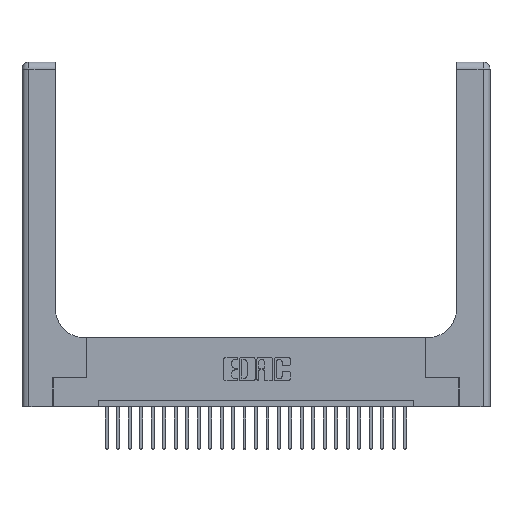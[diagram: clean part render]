
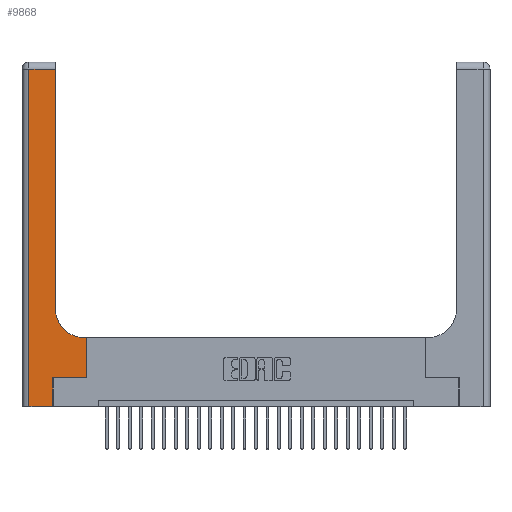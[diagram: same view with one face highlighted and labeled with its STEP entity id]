
A CAD part, top view. The second image highlights one B-rep face of the part: STEP entity #9868.
In plain terms, the highlighted planar face has unit normal (0, 0, 1).
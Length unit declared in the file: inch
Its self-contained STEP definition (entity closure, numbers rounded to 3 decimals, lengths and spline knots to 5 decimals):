
#436 = CARTESIAN_POINT ( 'NONE',  ( 0.2915, 3., 0.37 ) ) ;
#703 = DIRECTION ( 'NONE',  ( 1., 0., 0. ) ) ;
#1467 = VECTOR ( 'NONE', #26861, 39.37008 ) ;
#2086 = VECTOR ( 'NONE', #13174, 39.37008 ) ;
#2354 = CARTESIAN_POINT ( 'NONE',  ( 0.2915, 2.94, 0.37 ) ) ;
#2868 = ORIENTED_EDGE ( 'NONE', *, *, #5653, .T. ) ;
#3011 = LINE ( 'NONE', #5509, #11311 ) ;
#3412 = LINE ( 'NONE', #19778, #13361 ) ;
#3450 = LINE ( 'NONE', #25902, #2086 ) ;
#5258 = ORIENTED_EDGE ( 'NONE', *, *, #16077, .T. ) ;
#5509 = CARTESIAN_POINT ( 'NONE',  ( 0.5585, 0.25, 0.37 ) ) ;
#5653 = EDGE_CURVE ( 'NONE', #23626, #8141, #13226, .T. ) ;
#5696 = DIRECTION ( 'NONE',  ( 0., 0., -1. ) ) ;
#5724 = AXIS2_PLACEMENT_3D ( 'NONE', #27100, #14184, #27290 ) ;
#5874 = CARTESIAN_POINT ( 'NONE',  ( 0.5585, 0.6, 0.37 ) ) ;
#5972 = ORIENTED_EDGE ( 'NONE', *, *, #16115, .T. ) ;
#6153 = EDGE_CURVE ( 'NONE', #8141, #24420, #18216, .T. ) ;
#6887 = DIRECTION ( 'NONE',  ( 0., 1., 0. ) ) ;
#6962 = VERTEX_POINT ( 'NONE', #26243 ) ;
#7846 = CARTESIAN_POINT ( 'NONE',  ( 0., 2.94, 0.37 ) ) ;
#7862 = EDGE_LOOP ( 'NONE', ( #17325, #14913, #5258, #5972, #20539, #14708, #23998, #15144, #2868 ) ) ;
#8029 = CARTESIAN_POINT ( 'NONE',  ( 0.5415, 0.6, 0.37 ) ) ;
#8141 = VERTEX_POINT ( 'NONE', #10238 ) ;
#8987 = VECTOR ( 'NONE', #22697, 39.37008 ) ;
#9721 = VERTEX_POINT ( 'NONE', #13995 ) ;
#9868 = ADVANCED_FACE ( 'NONE', ( #16337 ), #20171, .F. ) ;
#9950 = CARTESIAN_POINT ( 'NONE',  ( 0.2915, 0.6, 0.37 ) ) ;
#10238 = CARTESIAN_POINT ( 'NONE',  ( 0.2915, 0.85, 0.37 ) ) ;
#10273 = EDGE_CURVE ( 'NONE', #9721, #6962, #3412, .T. ) ;
#11311 = VECTOR ( 'NONE', #22387, 39.37008 ) ;
#11412 = EDGE_CURVE ( 'NONE', #6962, #14732, #3011, .T. ) ;
#11796 = CARTESIAN_POINT ( 'NONE',  ( 0., 3., 0.37 ) ) ;
#11989 = DIRECTION ( 'NONE',  ( -1., 0., 0. ) ) ;
#12905 = AXIS2_PLACEMENT_3D ( 'NONE', #11796, #5696, #11989 ) ;
#13174 = DIRECTION ( 'NONE',  ( 0., -1., 0. ) ) ;
#13226 = CIRCLE ( 'NONE', #5724, 0.25 ) ;
#13361 = VECTOR ( 'NONE', #24047, 39.37008 ) ;
#13403 = VECTOR ( 'NONE', #703, 39.37008 ) ;
#13995 = CARTESIAN_POINT ( 'NONE',  ( 0.269, 0.25, 0.37 ) ) ;
#14184 = DIRECTION ( 'NONE',  ( 0., 0., -1. ) ) ;
#14266 = CARTESIAN_POINT ( 'NONE',  ( 0.269, 0., 0.37 ) ) ;
#14708 = ORIENTED_EDGE ( 'NONE', *, *, #10273, .T. ) ;
#14732 = VERTEX_POINT ( 'NONE', #5874 ) ;
#14913 = ORIENTED_EDGE ( 'NONE', *, *, #27536, .T. ) ;
#15122 = DIRECTION ( 'NONE',  ( 0., 1., 0. ) ) ;
#15144 = ORIENTED_EDGE ( 'NONE', *, *, #25613, .T. ) ;
#15391 = VERTEX_POINT ( 'NONE', #22232 ) ;
#16077 = EDGE_CURVE ( 'NONE', #15391, #21880, #3450, .T. ) ;
#16115 = EDGE_CURVE ( 'NONE', #21880, #23078, #19089, .T. ) ;
#16337 = FACE_OUTER_BOUND ( 'NONE', #7862, .T. ) ;
#16342 = LINE ( 'NONE', #7846, #8987 ) ;
#17325 = ORIENTED_EDGE ( 'NONE', *, *, #6153, .T. ) ;
#17888 = VECTOR ( 'NONE', #15122, 39.37008 ) ;
#18216 = LINE ( 'NONE', #436, #23180 ) ;
#18889 = EDGE_CURVE ( 'NONE', #23078, #9721, #22144, .T. ) ;
#19089 = LINE ( 'NONE', #19687, #13403 ) ;
#19687 = CARTESIAN_POINT ( 'NONE',  ( 0., 0., 0.37 ) ) ;
#19778 = CARTESIAN_POINT ( 'NONE',  ( 0.269, 0.25, 0.37 ) ) ;
#19932 = CARTESIAN_POINT ( 'NONE',  ( 0.06, 0., 0.37 ) ) ;
#20171 = PLANE ( 'NONE',  #12905 ) ;
#20539 = ORIENTED_EDGE ( 'NONE', *, *, #18889, .T. ) ;
#21416 = CARTESIAN_POINT ( 'NONE',  ( 0.269, 0., 0.37 ) ) ;
#21880 = VERTEX_POINT ( 'NONE', #19932 ) ;
#22144 = LINE ( 'NONE', #21416, #17888 ) ;
#22232 = CARTESIAN_POINT ( 'NONE',  ( 0.06, 2.94, 0.37 ) ) ;
#22387 = DIRECTION ( 'NONE',  ( 0., 1., 0. ) ) ;
#22697 = DIRECTION ( 'NONE',  ( -1., 0., 0. ) ) ;
#23078 = VERTEX_POINT ( 'NONE', #14266 ) ;
#23090 = LINE ( 'NONE', #9950, #1467 ) ;
#23180 = VECTOR ( 'NONE', #6887, 39.37008 ) ;
#23626 = VERTEX_POINT ( 'NONE', #8029 ) ;
#23998 = ORIENTED_EDGE ( 'NONE', *, *, #11412, .T. ) ;
#24047 = DIRECTION ( 'NONE',  ( 1., 0., 0. ) ) ;
#24420 = VERTEX_POINT ( 'NONE', #2354 ) ;
#25613 = EDGE_CURVE ( 'NONE', #14732, #23626, #23090, .T. ) ;
#25902 = CARTESIAN_POINT ( 'NONE',  ( 0.06, 3., 0.37 ) ) ;
#26243 = CARTESIAN_POINT ( 'NONE',  ( 0.5585, 0.25, 0.37 ) ) ;
#26861 = DIRECTION ( 'NONE',  ( -1., 0., 0. ) ) ;
#27100 = CARTESIAN_POINT ( 'NONE',  ( 0.5415, 0.85, 0.37 ) ) ;
#27290 = DIRECTION ( 'NONE',  ( 1., 0., 0. ) ) ;
#27536 = EDGE_CURVE ( 'NONE', #24420, #15391, #16342, .T. ) ;
